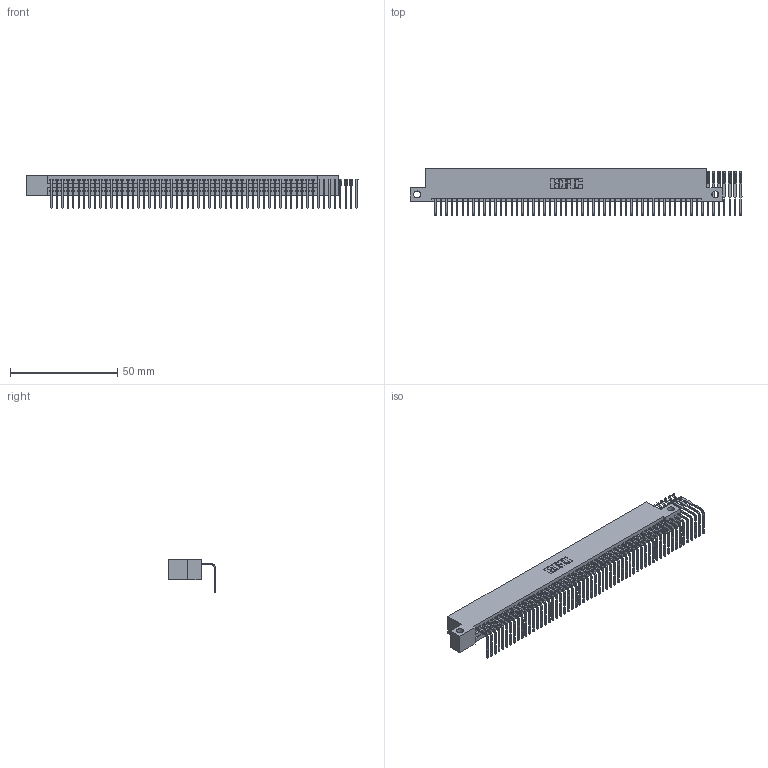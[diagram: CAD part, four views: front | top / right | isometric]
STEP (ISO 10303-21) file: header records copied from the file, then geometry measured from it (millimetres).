
FILE_DESCRIPTION (( 'STEP AP203' ), '1' );
FILE_NAME ('345-057-558-112.STEP', '2019-10-10T19:53:14', ( '' ), ( '' ), 'SwSTEP 2.0', 'SolidWorks 2016', '' );
FILE_SCHEMA (( 'CONFIG_CONTROL_DESIGN' ));
Length unit declared in the file: inch
Products named in the file (3): 345-057-558-112; 345 Part_Flush Mounting Lugs - Side Mount; 345-292-001_558 Tail - 2
Assembly tree (58 placements, depth 2):
  345-057-558-112
    345 Part_Flush Mounting Lugs - Side Mount
    345-292-001_558 Tail - 2  x57
Bounding box: 154.75 x 21.83 x 15.37 mm (x, y, z)
Volume: 14087.4 mm3; surface area: 20276.4 mm2
Topology: 58 solids, 58 shells, 3418 faces, 10283 edges, 6778 vertices
Faces by surface type: plane 2362, cylinder 1056
Entity records: 36279 total; most frequent: CARTESIAN_POINT 6255, ORIENTED_EDGE 6230, DIRECTION 5461, EDGE_CURVE 3115, VECTOR 2787, LINE 2787, VERTEX_POINT 2074, AXIS2_PLACEMENT_3D 1337
